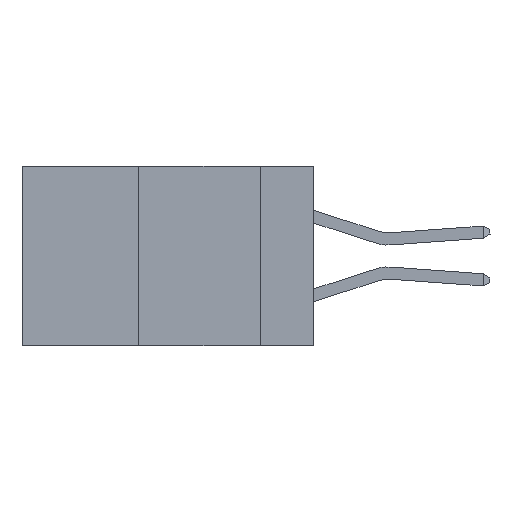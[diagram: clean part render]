
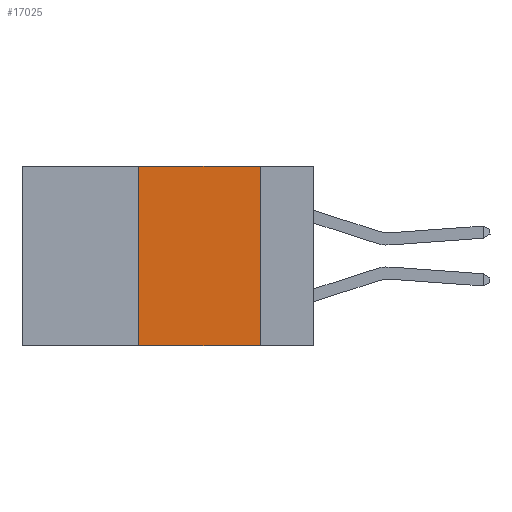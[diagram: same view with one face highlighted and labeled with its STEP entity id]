
A CAD part, left-side view. The second image highlights one B-rep face of the part: STEP entity #17025.
In plain terms, the highlighted planar face has unit normal (-1, 0, 0).
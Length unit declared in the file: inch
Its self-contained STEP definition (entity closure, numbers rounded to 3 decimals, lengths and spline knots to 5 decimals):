
#128 = FACE_OUTER_BOUND ( 'NONE', #1327, .T. ) ;
#1082 = CARTESIAN_POINT ( 'NONE',  ( 0., 0.11, 0. ) ) ;
#1327 = EDGE_LOOP ( 'NONE', ( #13562, #16039, #15899, #13839 ) ) ;
#2412 = CARTESIAN_POINT ( 'NONE',  ( 0., 0.6, 0. ) ) ;
#4751 = VERTEX_POINT ( 'NONE', #1082 ) ;
#8719 = VECTOR ( 'NONE', #25139, 39.37008 ) ;
#9451 = VECTOR ( 'NONE', #20834, 39.37008 ) ;
#11176 = DIRECTION ( 'NONE',  ( 1., 0., 0. ) ) ;
#11521 = EDGE_CURVE ( 'NONE', #21372, #4751, #27685, .T. ) ;
#12213 = AXIS2_PLACEMENT_3D ( 'NONE', #2412, #11176, #26022 ) ;
#13562 = ORIENTED_EDGE ( 'NONE', *, *, #22997, .F. ) ;
#13619 = LINE ( 'NONE', #24709, #24204 ) ;
#13839 = ORIENTED_EDGE ( 'NONE', *, *, #21445, .T. ) ;
#14296 = CARTESIAN_POINT ( 'NONE',  ( 0., 0.36, 0. ) ) ;
#15391 = VERTEX_POINT ( 'NONE', #20380 ) ;
#15419 = EDGE_CURVE ( 'NONE', #21131, #21372, #13619, .T. ) ;
#15899 = ORIENTED_EDGE ( 'NONE', *, *, #15419, .F. ) ;
#16039 = ORIENTED_EDGE ( 'NONE', *, *, #11521, .F. ) ;
#17025 = ADVANCED_FACE ( 'NONE', ( #128 ), #23892, .F. ) ;
#17926 = CARTESIAN_POINT ( 'NONE',  ( 0., 0.11, 0. ) ) ;
#18363 = DIRECTION ( 'NONE',  ( 0., 0., 1. ) ) ;
#18723 = CARTESIAN_POINT ( 'NONE',  ( 0., 0.6, -0.37 ) ) ;
#20380 = CARTESIAN_POINT ( 'NONE',  ( 0., 0.11, -0.37 ) ) ;
#20834 = DIRECTION ( 'NONE',  ( 0., -1., 0. ) ) ;
#21131 = VERTEX_POINT ( 'NONE', #24075 ) ;
#21372 = VERTEX_POINT ( 'NONE', #14296 ) ;
#21445 = EDGE_CURVE ( 'NONE', #21131, #15391, #25741, .T. ) ;
#22997 = EDGE_CURVE ( 'NONE', #4751, #15391, #25019, .T. ) ;
#23892 = PLANE ( 'NONE',  #12213 ) ;
#24075 = CARTESIAN_POINT ( 'NONE',  ( 0., 0.36, -0.37 ) ) ;
#24204 = VECTOR ( 'NONE', #18363, 39.37008 ) ;
#24709 = CARTESIAN_POINT ( 'NONE',  ( 0., 0.36, 0. ) ) ;
#25019 = LINE ( 'NONE', #17926, #8719 ) ;
#25139 = DIRECTION ( 'NONE',  ( 0., 0., -1. ) ) ;
#25419 = CARTESIAN_POINT ( 'NONE',  ( 0., 0.6, 0. ) ) ;
#25741 = LINE ( 'NONE', #18723, #9451 ) ;
#26022 = DIRECTION ( 'NONE',  ( 0., 0., -1. ) ) ;
#27038 = VECTOR ( 'NONE', #27557, 39.37008 ) ;
#27557 = DIRECTION ( 'NONE',  ( 0., -1., 0. ) ) ;
#27685 = LINE ( 'NONE', #25419, #27038 ) ;
